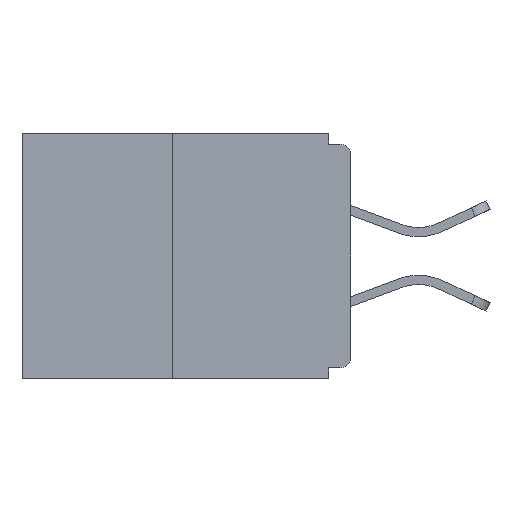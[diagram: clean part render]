
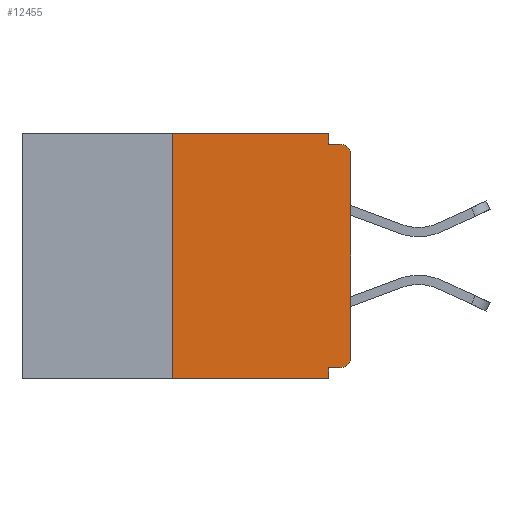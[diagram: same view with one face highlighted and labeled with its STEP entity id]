
A CAD part, left-side view. The second image highlights one B-rep face of the part: STEP entity #12455.
In plain terms, the highlighted planar face has unit normal (-1, 0, 0).
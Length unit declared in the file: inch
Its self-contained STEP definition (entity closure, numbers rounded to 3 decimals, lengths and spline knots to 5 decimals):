
#303 = ORIENTED_EDGE ( 'NONE', *, *, #7536, .T. ) ;
#757 = DIRECTION ( 'NONE',  ( 0., 1., 0. ) ) ;
#1228 = LINE ( 'NONE', #6588, #13914 ) ;
#1265 = LINE ( 'NONE', #15963, #8797 ) ;
#1425 = CARTESIAN_POINT ( 'NONE',  ( 0., 0.015, -0.03 ) ) ;
#1491 = CIRCLE ( 'NONE', #11270, 0.015 ) ;
#1669 = ORIENTED_EDGE ( 'NONE', *, *, #9654, .F. ) ;
#1880 = PLANE ( 'NONE',  #15198 ) ;
#2247 = LINE ( 'NONE', #12762, #15880 ) ;
#2488 = ORIENTED_EDGE ( 'NONE', *, *, #16781, .F. ) ;
#2497 = EDGE_CURVE ( 'NONE', #10976, #8587, #2675, .T. ) ;
#2592 = LINE ( 'NONE', #5128, #9047 ) ;
#2675 = CIRCLE ( 'NONE', #16649, 0.015 ) ;
#3092 = DIRECTION ( 'NONE',  ( 0., 0., -1. ) ) ;
#3533 = VERTEX_POINT ( 'NONE', #10344 ) ;
#3568 = EDGE_CURVE ( 'NONE', #12233, #10976, #1228, .T. ) ;
#4047 = DIRECTION ( 'NONE',  ( 0., 0., -1. ) ) ;
#4063 = ORIENTED_EDGE ( 'NONE', *, *, #6601, .F. ) ;
#4545 = VECTOR ( 'NONE', #10957, 39.37008 ) ;
#4966 = EDGE_CURVE ( 'NONE', #7698, #14891, #2247, .T. ) ;
#5128 = CARTESIAN_POINT ( 'NONE',  ( 0., 0.46, -0.343 ) ) ;
#6364 = CARTESIAN_POINT ( 'NONE',  ( 0., 0.46, 0. ) ) ;
#6469 = ORIENTED_EDGE ( 'NONE', *, *, #7541, .T. ) ;
#6588 = CARTESIAN_POINT ( 'NONE',  ( 0., 0., 0. ) ) ;
#6601 = EDGE_CURVE ( 'NONE', #8936, #8587, #15018, .T. ) ;
#6962 = VERTEX_POINT ( 'NONE', #7355 ) ;
#7324 = CARTESIAN_POINT ( 'NONE',  ( 0., 0., -0.313 ) ) ;
#7355 = CARTESIAN_POINT ( 'NONE',  ( 0., 0.25, 0. ) ) ;
#7536 = EDGE_CURVE ( 'NONE', #11614, #9357, #2592, .T. ) ;
#7541 = EDGE_CURVE ( 'NONE', #7698, #12233, #1491, .T. ) ;
#7698 = VERTEX_POINT ( 'NONE', #12543 ) ;
#8202 = ORIENTED_EDGE ( 'NONE', *, *, #16125, .F. ) ;
#8212 = VECTOR ( 'NONE', #17019, 39.37008 ) ;
#8272 = CARTESIAN_POINT ( 'NONE',  ( 0., 0., -0.03 ) ) ;
#8587 = VERTEX_POINT ( 'NONE', #12325 ) ;
#8797 = VECTOR ( 'NONE', #9241, 39.37008 ) ;
#8936 = VERTEX_POINT ( 'NONE', #10605 ) ;
#9047 = VECTOR ( 'NONE', #13378, 39.37008 ) ;
#9153 = ORIENTED_EDGE ( 'NONE', *, *, #3568, .T. ) ;
#9241 = DIRECTION ( 'NONE',  ( 0., 0., -1. ) ) ;
#9272 = ORIENTED_EDGE ( 'NONE', *, *, #4966, .F. ) ;
#9357 = VERTEX_POINT ( 'NONE', #14600 ) ;
#9587 = DIRECTION ( 'NONE',  ( 0., 0., -1. ) ) ;
#9654 = EDGE_CURVE ( 'NONE', #6962, #3533, #16759, .T. ) ;
#9870 = CARTESIAN_POINT ( 'NONE',  ( 0., 0., -0.015 ) ) ;
#10344 = CARTESIAN_POINT ( 'NONE',  ( 0., 0.031, 0. ) ) ;
#10605 = CARTESIAN_POINT ( 'NONE',  ( 0., 0.031, -0.015 ) ) ;
#10957 = DIRECTION ( 'NONE',  ( 0., 0., 1. ) ) ;
#10976 = VERTEX_POINT ( 'NONE', #8272 ) ;
#11270 = AXIS2_PLACEMENT_3D ( 'NONE', #14520, #17105, #15982 ) ;
#11614 = VERTEX_POINT ( 'NONE', #14971 ) ;
#12233 = VERTEX_POINT ( 'NONE', #7324 ) ;
#12299 = DIRECTION ( 'NONE',  ( 1., 0., 0. ) ) ;
#12325 = CARTESIAN_POINT ( 'NONE',  ( 0., 0.015, -0.015 ) ) ;
#12344 = CARTESIAN_POINT ( 'NONE',  ( 0., 0.25, 0. ) ) ;
#12455 = ADVANCED_FACE ( 'NONE', ( #16415 ), #1880, .F. ) ;
#12543 = CARTESIAN_POINT ( 'NONE',  ( 0., 0.015, -0.328 ) ) ;
#12620 = LINE ( 'NONE', #13616, #13828 ) ;
#12762 = CARTESIAN_POINT ( 'NONE',  ( 0., 0., -0.328 ) ) ;
#12836 = ORIENTED_EDGE ( 'NONE', *, *, #17203, .F. ) ;
#13378 = DIRECTION ( 'NONE',  ( 0., -1., 0. ) ) ;
#13616 = CARTESIAN_POINT ( 'NONE',  ( 0., 0.031, 0. ) ) ;
#13828 = VECTOR ( 'NONE', #9587, 39.37008 ) ;
#13914 = VECTOR ( 'NONE', #15940, 39.37008 ) ;
#14520 = CARTESIAN_POINT ( 'NONE',  ( 0., 0.015, -0.313 ) ) ;
#14530 = EDGE_LOOP ( 'NONE', ( #1669, #8202, #303, #2488, #9272, #6469, #9153, #16461, #4063, #12836 ) ) ;
#14600 = CARTESIAN_POINT ( 'NONE',  ( 0., 0.031, -0.343 ) ) ;
#14891 = VERTEX_POINT ( 'NONE', #15637 ) ;
#14971 = CARTESIAN_POINT ( 'NONE',  ( 0., 0.25, -0.343 ) ) ;
#15018 = LINE ( 'NONE', #9870, #15539 ) ;
#15172 = CARTESIAN_POINT ( 'NONE',  ( 0., 0.46, 0. ) ) ;
#15198 = AXIS2_PLACEMENT_3D ( 'NONE', #15172, #12299, #3092 ) ;
#15539 = VECTOR ( 'NONE', #16501, 39.37008 ) ;
#15637 = CARTESIAN_POINT ( 'NONE',  ( 0., 0.031, -0.328 ) ) ;
#15880 = VECTOR ( 'NONE', #757, 39.37008 ) ;
#15940 = DIRECTION ( 'NONE',  ( 0., 0., 1. ) ) ;
#15963 = CARTESIAN_POINT ( 'NONE',  ( 0., 0.031, -0.343 ) ) ;
#15982 = DIRECTION ( 'NONE',  ( 0., 0., -1. ) ) ;
#16125 = EDGE_CURVE ( 'NONE', #11614, #6962, #16468, .T. ) ;
#16415 = FACE_OUTER_BOUND ( 'NONE', #14530, .T. ) ;
#16461 = ORIENTED_EDGE ( 'NONE', *, *, #2497, .T. ) ;
#16468 = LINE ( 'NONE', #12344, #4545 ) ;
#16501 = DIRECTION ( 'NONE',  ( 0., -1., 0. ) ) ;
#16649 = AXIS2_PLACEMENT_3D ( 'NONE', #1425, #17265, #4047 ) ;
#16759 = LINE ( 'NONE', #6364, #8212 ) ;
#16781 = EDGE_CURVE ( 'NONE', #14891, #9357, #1265, .T. ) ;
#17019 = DIRECTION ( 'NONE',  ( 0., -1., 0. ) ) ;
#17105 = DIRECTION ( 'NONE',  ( -1., 0., 0. ) ) ;
#17203 = EDGE_CURVE ( 'NONE', #3533, #8936, #12620, .T. ) ;
#17265 = DIRECTION ( 'NONE',  ( -1., 0., 0. ) ) ;
